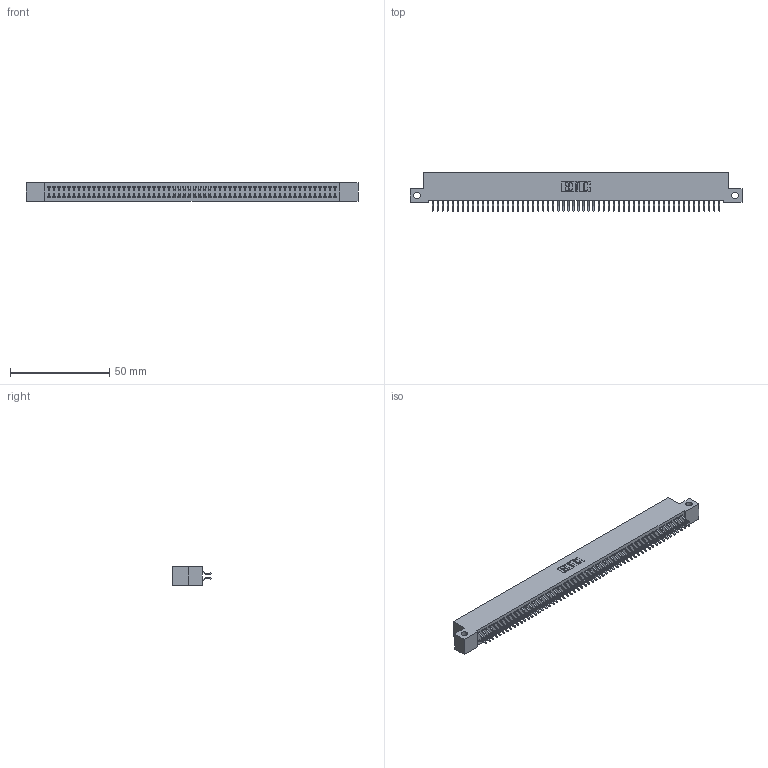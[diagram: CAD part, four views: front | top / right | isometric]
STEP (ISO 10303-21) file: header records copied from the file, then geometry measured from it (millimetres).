
FILE_DESCRIPTION (( 'STEP AP203' ), '1' );
FILE_NAME ('392-116-556-212.STEP', '2019-10-10T01:59:24', ( '' ), ( '' ), 'SwSTEP 2.0', 'SolidWorks 2016', '' );
FILE_SCHEMA (( 'CONFIG_CONTROL_DESIGN' ));
Length unit declared in the file: inch
Products named in the file (3): 342 Part_Side Mount; 345-292-001_556 Tail; 392-116-556-212
Assembly tree (117 placements, depth 2):
  392-116-556-212
    342 Part_Side Mount
    345-292-001_556 Tail  x116
Bounding box: 167.64 x 19.58 x 9.4 mm (x, y, z)
Volume: 15061.3 mm3; surface area: 24638 mm2
Topology: 117 solids, 117 shells, 6838 faces, 20367 edges, 13422 vertices
Faces by surface type: plane 4706, cylinder 2132
Entity records: 35335 total; most frequent: CARTESIAN_POINT 5850, ORIENTED_EDGE 5774, DIRECTION 4959, EDGE_CURVE 2887, LINE 2751, VECTOR 2751, VERTEX_POINT 1922, AXIS2_PLACEMENT_3D 1104
